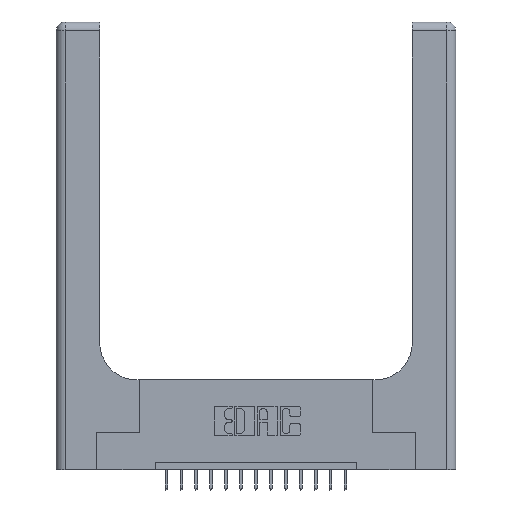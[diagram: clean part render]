
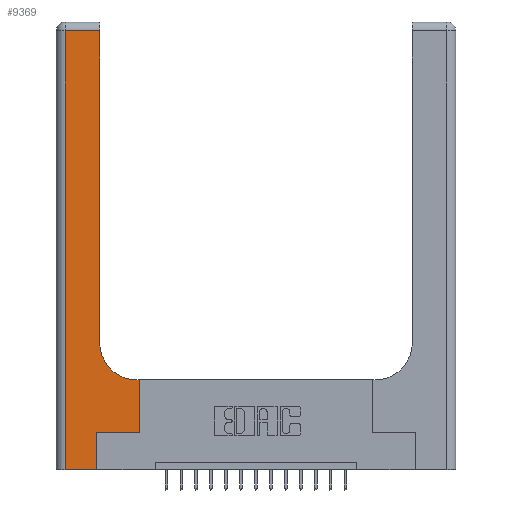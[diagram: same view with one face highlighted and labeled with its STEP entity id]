
A CAD part, top view. The second image highlights one B-rep face of the part: STEP entity #9369.
In plain terms, the highlighted planar face has unit normal (0, 0, 1).
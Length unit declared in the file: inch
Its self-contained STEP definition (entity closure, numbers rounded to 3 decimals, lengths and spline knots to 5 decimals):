
#22 = VECTOR ( 'NONE', #4250, 39.37008 ) ;
#309 = CARTESIAN_POINT ( 'NONE',  ( 0.269, 0.25, 0.37 ) ) ;
#410 = CARTESIAN_POINT ( 'NONE',  ( 0.5585, 0.25, 0.37 ) ) ;
#1020 = VECTOR ( 'NONE', #7627, 39.37008 ) ;
#1318 = LINE ( 'NONE', #2762, #18448 ) ;
#1444 = ORIENTED_EDGE ( 'NONE', *, *, #1658, .T. ) ;
#1658 = EDGE_CURVE ( 'NONE', #3647, #3411, #3612, .T. ) ;
#1890 = DIRECTION ( 'NONE',  ( 0., 1., 0. ) ) ;
#1969 = DIRECTION ( 'NONE',  ( 0., 0., -1. ) ) ;
#2014 = CARTESIAN_POINT ( 'NONE',  ( 0.06, 3., 0.37 ) ) ;
#2637 = LINE ( 'NONE', #18730, #10563 ) ;
#2762 = CARTESIAN_POINT ( 'NONE',  ( 0.269, 0.25, 0.37 ) ) ;
#3107 = VERTEX_POINT ( 'NONE', #18355 ) ;
#3216 = LINE ( 'NONE', #410, #1020 ) ;
#3278 = LINE ( 'NONE', #2014, #9002 ) ;
#3292 = DIRECTION ( 'NONE',  ( 0., 0., -1. ) ) ;
#3348 = CARTESIAN_POINT ( 'NONE',  ( 0.06, 0., 0.37 ) ) ;
#3411 = VERTEX_POINT ( 'NONE', #14893 ) ;
#3436 = LINE ( 'NONE', #14853, #14549 ) ;
#3612 = CIRCLE ( 'NONE', #9755, 0.25 ) ;
#3647 = VERTEX_POINT ( 'NONE', #4808 ) ;
#3957 = EDGE_LOOP ( 'NONE', ( #14229, #4061, #8870, #10021, #7410, #11119, #12533, #16626, #1444 ) ) ;
#4061 = ORIENTED_EDGE ( 'NONE', *, *, #6485, .T. ) ;
#4250 = DIRECTION ( 'NONE',  ( -1., 0., 0. ) ) ;
#4331 = VERTEX_POINT ( 'NONE', #16484 ) ;
#4808 = CARTESIAN_POINT ( 'NONE',  ( 0.5415, 0.6, 0.37 ) ) ;
#5881 = CARTESIAN_POINT ( 'NONE',  ( 0., 2.94, 0.37 ) ) ;
#6485 = EDGE_CURVE ( 'NONE', #3107, #4331, #9999, .T. ) ;
#6904 = VERTEX_POINT ( 'NONE', #16965 ) ;
#7410 = ORIENTED_EDGE ( 'NONE', *, *, #12140, .T. ) ;
#7627 = DIRECTION ( 'NONE',  ( 0., 1., 0. ) ) ;
#7677 = DIRECTION ( 'NONE',  ( -1., 0., 0. ) ) ;
#7708 = CARTESIAN_POINT ( 'NONE',  ( 0.5415, 0.85, 0.37 ) ) ;
#8870 = ORIENTED_EDGE ( 'NONE', *, *, #16664, .T. ) ;
#9002 = VECTOR ( 'NONE', #12108, 39.37008 ) ;
#9008 = CARTESIAN_POINT ( 'NONE',  ( 0.2915, 3., 0.37 ) ) ;
#9176 = FACE_OUTER_BOUND ( 'NONE', #3957, .T. ) ;
#9369 = ADVANCED_FACE ( 'NONE', ( #9176 ), #12050, .F. ) ;
#9755 = AXIS2_PLACEMENT_3D ( 'NONE', #7708, #3292, #13169 ) ;
#9999 = LINE ( 'NONE', #5881, #22 ) ;
#10021 = ORIENTED_EDGE ( 'NONE', *, *, #14624, .T. ) ;
#10513 = DIRECTION ( 'NONE',  ( -1., 0., 0. ) ) ;
#10563 = VECTOR ( 'NONE', #15500, 39.37008 ) ;
#10798 = CARTESIAN_POINT ( 'NONE',  ( 0., 3., 0.37 ) ) ;
#11019 = EDGE_CURVE ( 'NONE', #12622, #12854, #3216, .T. ) ;
#11087 = DIRECTION ( 'NONE',  ( 1., 0., 0. ) ) ;
#11119 = ORIENTED_EDGE ( 'NONE', *, *, #12754, .T. ) ;
#12050 = PLANE ( 'NONE',  #18773 ) ;
#12059 = VECTOR ( 'NONE', #11087, 39.37008 ) ;
#12108 = DIRECTION ( 'NONE',  ( 0., -1., 0. ) ) ;
#12140 = EDGE_CURVE ( 'NONE', #6904, #17562, #2637, .T. ) ;
#12533 = ORIENTED_EDGE ( 'NONE', *, *, #11019, .T. ) ;
#12622 = VERTEX_POINT ( 'NONE', #15525 ) ;
#12754 = EDGE_CURVE ( 'NONE', #17562, #12622, #1318, .T. ) ;
#12854 = VERTEX_POINT ( 'NONE', #14745 ) ;
#12929 = EDGE_CURVE ( 'NONE', #3411, #3107, #16276, .T. ) ;
#13169 = DIRECTION ( 'NONE',  ( 1., 0., 0. ) ) ;
#13666 = LINE ( 'NONE', #13755, #12059 ) ;
#13755 = CARTESIAN_POINT ( 'NONE',  ( 0., 0., 0.37 ) ) ;
#14229 = ORIENTED_EDGE ( 'NONE', *, *, #12929, .T. ) ;
#14549 = VECTOR ( 'NONE', #7677, 39.37008 ) ;
#14624 = EDGE_CURVE ( 'NONE', #18501, #6904, #13666, .T. ) ;
#14745 = CARTESIAN_POINT ( 'NONE',  ( 0.5585, 0.6, 0.37 ) ) ;
#14853 = CARTESIAN_POINT ( 'NONE',  ( 0.2915, 0.6, 0.37 ) ) ;
#14893 = CARTESIAN_POINT ( 'NONE',  ( 0.2915, 0.85, 0.37 ) ) ;
#15500 = DIRECTION ( 'NONE',  ( 0., 1., 0. ) ) ;
#15525 = CARTESIAN_POINT ( 'NONE',  ( 0.5585, 0.25, 0.37 ) ) ;
#15807 = DIRECTION ( 'NONE',  ( 1., 0., 0. ) ) ;
#16276 = LINE ( 'NONE', #9008, #18742 ) ;
#16484 = CARTESIAN_POINT ( 'NONE',  ( 0.06, 2.94, 0.37 ) ) ;
#16626 = ORIENTED_EDGE ( 'NONE', *, *, #18409, .T. ) ;
#16664 = EDGE_CURVE ( 'NONE', #4331, #18501, #3278, .T. ) ;
#16965 = CARTESIAN_POINT ( 'NONE',  ( 0.269, 0., 0.37 ) ) ;
#17562 = VERTEX_POINT ( 'NONE', #309 ) ;
#18355 = CARTESIAN_POINT ( 'NONE',  ( 0.2915, 2.94, 0.37 ) ) ;
#18409 = EDGE_CURVE ( 'NONE', #12854, #3647, #3436, .T. ) ;
#18448 = VECTOR ( 'NONE', #15807, 39.37008 ) ;
#18501 = VERTEX_POINT ( 'NONE', #3348 ) ;
#18730 = CARTESIAN_POINT ( 'NONE',  ( 0.269, 0., 0.37 ) ) ;
#18742 = VECTOR ( 'NONE', #1890, 39.37008 ) ;
#18773 = AXIS2_PLACEMENT_3D ( 'NONE', #10798, #1969, #10513 ) ;
